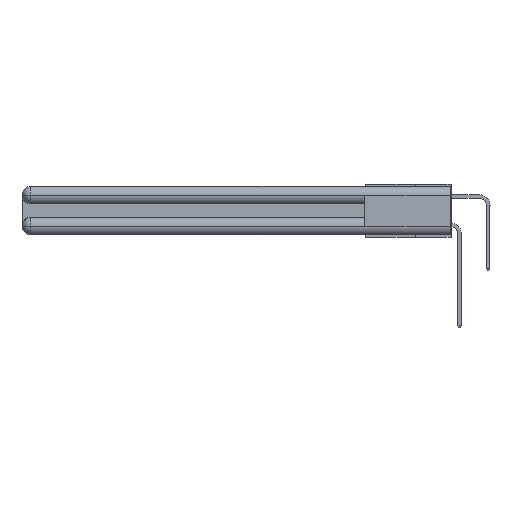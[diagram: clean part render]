
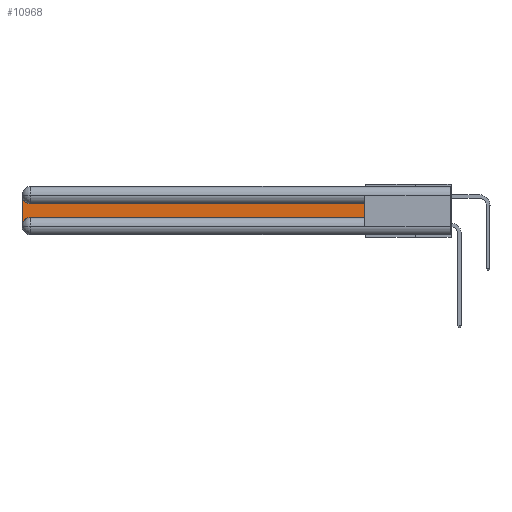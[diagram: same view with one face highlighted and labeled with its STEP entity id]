
A CAD part, left-side view. The second image highlights one B-rep face of the part: STEP entity #10968.
In plain terms, the highlighted planar face has unit normal (-1, 0, 0).
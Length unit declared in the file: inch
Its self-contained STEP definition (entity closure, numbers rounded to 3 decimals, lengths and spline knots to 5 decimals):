
#226 = DIRECTION ( 'NONE',  ( 0., 0., -1. ) ) ;
#1016 = ORIENTED_EDGE ( 'NONE', *, *, #11421, .T. ) ;
#2807 = CARTESIAN_POINT ( 'NONE',  ( 0.075, 3., -0.1225 ) ) ;
#3219 = DIRECTION ( 'NONE',  ( 0., 0., -1. ) ) ;
#4194 = CARTESIAN_POINT ( 'NONE',  ( 0.075, 2.94, -0.2175 ) ) ;
#4839 = LINE ( 'NONE', #15961, #31880 ) ;
#5442 = DIRECTION ( 'NONE',  ( 1., 0., 0. ) ) ;
#6231 = ORIENTED_EDGE ( 'NONE', *, *, #26731, .T. ) ;
#6573 = EDGE_CURVE ( 'NONE', #6669, #13913, #21755, .T. ) ;
#6669 = VERTEX_POINT ( 'NONE', #29879 ) ;
#7524 = CARTESIAN_POINT ( 'NONE',  ( 0.075, 0.6, -0.2175 ) ) ;
#7829 = ORIENTED_EDGE ( 'NONE', *, *, #32413, .T. ) ;
#7926 = FACE_OUTER_BOUND ( 'NONE', #13631, .T. ) ;
#8351 = EDGE_CURVE ( 'NONE', #33165, #6669, #4839, .T. ) ;
#8855 = DIRECTION ( 'NONE',  ( 0., 0., 1. ) ) ;
#9209 = CARTESIAN_POINT ( 'NONE',  ( 0.075, 3., -0.0625 ) ) ;
#9890 = VERTEX_POINT ( 'NONE', #7524 ) ;
#10007 = CARTESIAN_POINT ( 'NONE',  ( 0.075, 0.6, -0.2175 ) ) ;
#10264 = ORIENTED_EDGE ( 'NONE', *, *, #6573, .T. ) ;
#10716 = DIRECTION ( 'NONE',  ( 0., 1., 0. ) ) ;
#10968 = ADVANCED_FACE ( 'NONE', ( #7926 ), #18499, .F. ) ;
#11142 = DIRECTION ( 'NONE',  ( 1., 0., 0. ) ) ;
#11421 = EDGE_CURVE ( 'NONE', #15767, #9890, #18131, .T. ) ;
#11802 = AXIS2_PLACEMENT_3D ( 'NONE', #18085, #11142, #3219 ) ;
#12425 = VECTOR ( 'NONE', #20480, 39.37008 ) ;
#12877 = AXIS2_PLACEMENT_3D ( 'NONE', #2807, #5442, #28775 ) ;
#13334 = VERTEX_POINT ( 'NONE', #29127 ) ;
#13631 = EDGE_LOOP ( 'NONE', ( #19508, #10264, #6231, #7829, #1016, #25823 ) ) ;
#13913 = VERTEX_POINT ( 'NONE', #9209 ) ;
#15767 = VERTEX_POINT ( 'NONE', #4194 ) ;
#15883 = DIRECTION ( 'NONE',  ( 1., 0., 0. ) ) ;
#15961 = CARTESIAN_POINT ( 'NONE',  ( 0.075, 0.6, -0.1225 ) ) ;
#17443 = AXIS2_PLACEMENT_3D ( 'NONE', #31535, #15883, #226 ) ;
#18085 = CARTESIAN_POINT ( 'NONE',  ( 0.075, 2.94, -0.0625 ) ) ;
#18131 = LINE ( 'NONE', #10007, #12425 ) ;
#18499 = PLANE ( 'NONE',  #12877 ) ;
#18662 = EDGE_CURVE ( 'NONE', #9890, #33165, #31922, .T. ) ;
#19508 = ORIENTED_EDGE ( 'NONE', *, *, #8351, .T. ) ;
#19739 = CARTESIAN_POINT ( 'NONE',  ( 0.075, 3., -0.2175 ) ) ;
#20480 = DIRECTION ( 'NONE',  ( 0., -1., 0. ) ) ;
#21673 = VECTOR ( 'NONE', #8855, 39.37008 ) ;
#21755 = CIRCLE ( 'NONE', #11802, 0.06 ) ;
#22129 = DIRECTION ( 'NONE',  ( 0., 0., -1. ) ) ;
#24186 = CARTESIAN_POINT ( 'NONE',  ( 0.075, 0.6, -0.1225 ) ) ;
#25823 = ORIENTED_EDGE ( 'NONE', *, *, #18662, .T. ) ;
#26731 = EDGE_CURVE ( 'NONE', #13913, #13334, #29000, .T. ) ;
#27001 = CARTESIAN_POINT ( 'NONE',  ( 0.075, 0.6, -0.2175 ) ) ;
#28775 = DIRECTION ( 'NONE',  ( 0., 0., -1. ) ) ;
#29000 = LINE ( 'NONE', #19739, #30624 ) ;
#29127 = CARTESIAN_POINT ( 'NONE',  ( 0.075, 3., -0.2775 ) ) ;
#29746 = CIRCLE ( 'NONE', #17443, 0.06 ) ;
#29879 = CARTESIAN_POINT ( 'NONE',  ( 0.075, 2.94, -0.1225 ) ) ;
#30624 = VECTOR ( 'NONE', #22129, 39.37008 ) ;
#31535 = CARTESIAN_POINT ( 'NONE',  ( 0.075, 2.94, -0.2775 ) ) ;
#31880 = VECTOR ( 'NONE', #10716, 39.37008 ) ;
#31922 = LINE ( 'NONE', #27001, #21673 ) ;
#32413 = EDGE_CURVE ( 'NONE', #13334, #15767, #29746, .T. ) ;
#33165 = VERTEX_POINT ( 'NONE', #24186 ) ;
